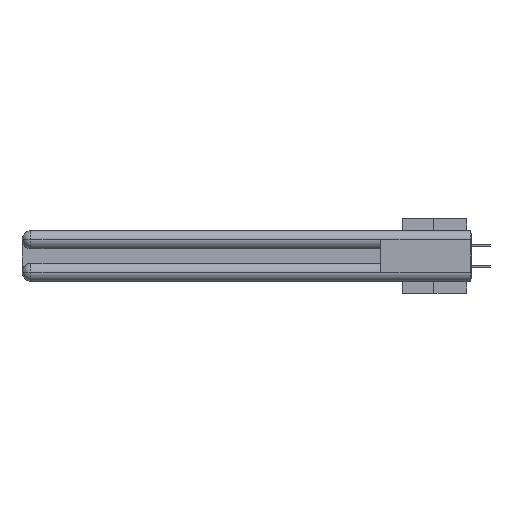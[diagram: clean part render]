
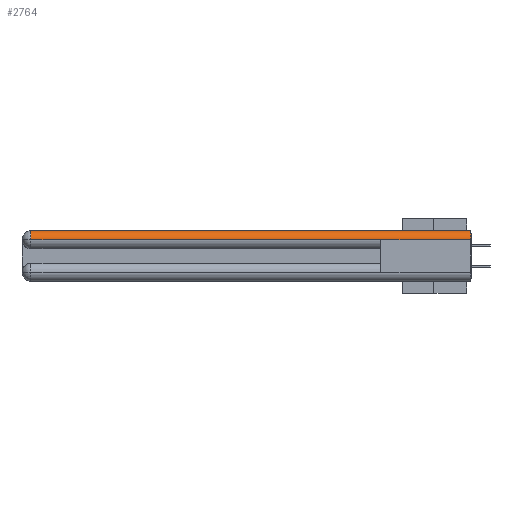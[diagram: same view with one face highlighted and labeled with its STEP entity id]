
A CAD part, left-side view. The second image highlights one B-rep face of the part: STEP entity #2764.
In plain terms, the highlighted cylindrical face has radius 1.562 mm (diameter 3.124 mm), a partial arc.
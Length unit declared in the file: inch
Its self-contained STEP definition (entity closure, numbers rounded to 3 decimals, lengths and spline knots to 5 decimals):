
#1926 = LINE ( 'NONE', #40204, #21612 ) ;
#2247 = CARTESIAN_POINT ( 'NONE',  ( 0.0615, 2.94, 0. ) ) ;
#2764 = ADVANCED_FACE ( 'NONE', ( #8196 ), #41191, .T. ) ;
#4297 = ORIENTED_EDGE ( 'NONE', *, *, #32593, .F. ) ;
#5375 = EDGE_CURVE ( 'NONE', #23068, #43059, #6892, .T. ) ;
#5687 = ORIENTED_EDGE ( 'NONE', *, *, #23631, .F. ) ;
#5895 = CARTESIAN_POINT ( 'NONE',  ( 0.0615, 0., 0. ) ) ;
#6892 = LINE ( 'NONE', #17956, #45095 ) ;
#8196 = FACE_OUTER_BOUND ( 'NONE', #42279, .T. ) ;
#12068 = CARTESIAN_POINT ( 'NONE',  ( 0., 0., -0.0615 ) ) ;
#12731 = AXIS2_PLACEMENT_3D ( 'NONE', #42903, #38885, #20582 ) ;
#14072 = DIRECTION ( 'NONE',  ( 0., -1., 0. ) ) ;
#14163 = DIRECTION ( 'NONE',  ( 0., -1., 0. ) ) ;
#14397 = DIRECTION ( 'NONE',  ( 0., 1., 0. ) ) ;
#17154 = DIRECTION ( 'NONE',  ( 0., 1., 0. ) ) ;
#17956 = CARTESIAN_POINT ( 'NONE',  ( 0., 3., -0.0615 ) ) ;
#18170 = CARTESIAN_POINT ( 'NONE',  ( 0., 0.6, -0.0615 ) ) ;
#19544 = CIRCLE ( 'NONE', #28815, 0.0615 ) ;
#19917 = VECTOR ( 'NONE', #14397, 39.37008 ) ;
#20582 = DIRECTION ( 'NONE',  ( 0., 0., 1. ) ) ;
#20850 = DIRECTION ( 'NONE',  ( 0., 0., 1. ) ) ;
#21576 = CARTESIAN_POINT ( 'NONE',  ( 0.0615, 0., -0.0615 ) ) ;
#21612 = VECTOR ( 'NONE', #14163, 39.37008 ) ;
#23068 = VERTEX_POINT ( 'NONE', #25694 ) ;
#23631 = EDGE_CURVE ( 'NONE', #26665, #24538, #19544, .T. ) ;
#24009 = EDGE_CURVE ( 'NONE', #42035, #23068, #29311, .T. ) ;
#24538 = VERTEX_POINT ( 'NONE', #12068 ) ;
#25630 = EDGE_CURVE ( 'NONE', #24538, #43059, #39623, .T. ) ;
#25694 = CARTESIAN_POINT ( 'NONE',  ( 0., 2.94, -0.0615 ) ) ;
#26665 = VERTEX_POINT ( 'NONE', #5895 ) ;
#28159 = AXIS2_PLACEMENT_3D ( 'NONE', #35470, #17154, #20850 ) ;
#28815 = AXIS2_PLACEMENT_3D ( 'NONE', #21576, #29024, #44391 ) ;
#29024 = DIRECTION ( 'NONE',  ( 0., -1., 0. ) ) ;
#29311 = CIRCLE ( 'NONE', #12731, 0.0615 ) ;
#32593 = EDGE_CURVE ( 'NONE', #42035, #26665, #1926, .T. ) ;
#34066 = ORIENTED_EDGE ( 'NONE', *, *, #25630, .F. ) ;
#35470 = CARTESIAN_POINT ( 'NONE',  ( 0.0615, 0., -0.0615 ) ) ;
#36477 = ORIENTED_EDGE ( 'NONE', *, *, #24009, .T. ) ;
#37049 = CARTESIAN_POINT ( 'NONE',  ( 0., 3., -0.0615 ) ) ;
#38339 = ORIENTED_EDGE ( 'NONE', *, *, #5375, .T. ) ;
#38885 = DIRECTION ( 'NONE',  ( 0., -1., 0. ) ) ;
#39623 = LINE ( 'NONE', #37049, #19917 ) ;
#40204 = CARTESIAN_POINT ( 'NONE',  ( 0.0615, 0., 0. ) ) ;
#41191 = CYLINDRICAL_SURFACE ( 'NONE', #28159, 0.0615 ) ;
#42035 = VERTEX_POINT ( 'NONE', #2247 ) ;
#42279 = EDGE_LOOP ( 'NONE', ( #4297, #36477, #38339, #34066, #5687 ) ) ;
#42903 = CARTESIAN_POINT ( 'NONE',  ( 0.0615, 2.94, -0.0615 ) ) ;
#43059 = VERTEX_POINT ( 'NONE', #18170 ) ;
#44391 = DIRECTION ( 'NONE',  ( 1., 0., 0. ) ) ;
#45095 = VECTOR ( 'NONE', #14072, 39.37008 ) ;
